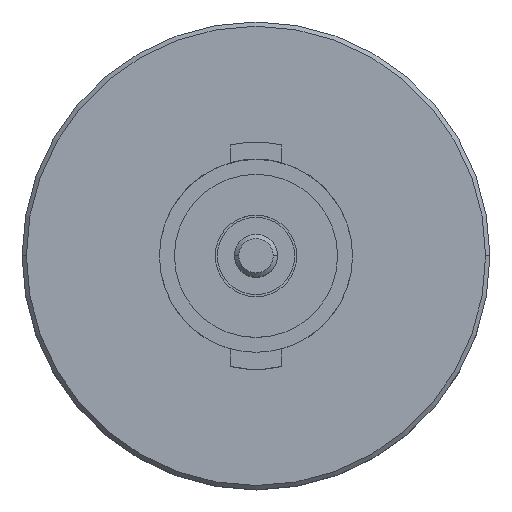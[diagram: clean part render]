
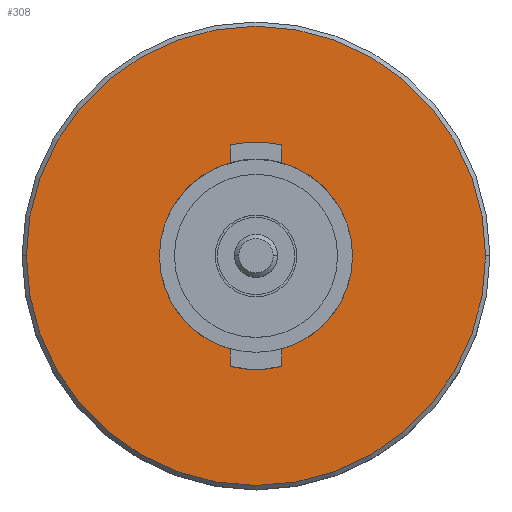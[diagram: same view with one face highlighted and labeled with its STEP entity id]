
A CAD part, top view. The second image highlights one B-rep face of the part: STEP entity #308.
In plain terms, the highlighted planar face has unit normal (0, 0, 1).
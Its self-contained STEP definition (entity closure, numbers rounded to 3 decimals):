
#24 = VECTOR ( 'NONE', #396, 1000. ) ;
#30 = DIRECTION ( 'NONE',  ( 0., 0., 1. ) ) ;
#41 = EDGE_CURVE ( 'NONE', #1158, #607, #622, .T. ) ;
#80 = AXIS2_PLACEMENT_3D ( 'NONE', #1608, #30, #760 ) ;
#83 = ORIENTED_EDGE ( 'NONE', *, *, #1763, .F. ) ;
#91 = CIRCLE ( 'NONE', #80, 2.25 ) ;
#105 = DIRECTION ( 'NONE',  ( -0.267, 0.964, 0. ) ) ;
#125 = AXIS2_PLACEMENT_3D ( 'NONE', #387, #1079, #1749 ) ;
#137 = EDGE_CURVE ( 'NONE', #607, #1485, #1885, .T. ) ;
#153 = VERTEX_POINT ( 'NONE', #1266 ) ;
#205 = CIRCLE ( 'NONE', #125, 2.25 ) ;
#216 = AXIS2_PLACEMENT_3D ( 'NONE', #491, #1185, #1853 ) ;
#240 = CARTESIAN_POINT ( 'NONE',  ( 20., 0., 30. ) ) ;
#242 = LINE ( 'NONE', #950, #2121 ) ;
#244 = EDGE_CURVE ( 'NONE', #1871, #1463, #91, .T. ) ;
#308 = ADVANCED_FACE ( 'NONE', ( #430, #1120 ), #1789, .T. ) ;
#329 = DIRECTION ( 'NONE',  ( -1., 0., 0. ) ) ;
#339 = AXIS2_PLACEMENT_3D ( 'NONE', #240, #948, #1626 ) ;
#360 = CARTESIAN_POINT ( 'NONE',  ( 19.4, 2.581, 30. ) ) ;
#381 = ORIENTED_EDGE ( 'NONE', *, *, #2131, .F. ) ;
#387 = CARTESIAN_POINT ( 'NONE',  ( 20., 0., 30. ) ) ;
#396 = DIRECTION ( 'NONE',  ( 0., -1., 0. ) ) ;
#401 = DIRECTION ( 'NONE',  ( 0., 0., 1. ) ) ;
#430 = FACE_OUTER_BOUND ( 'NONE', #1325, .T. ) ;
#490 = CARTESIAN_POINT ( 'NONE',  ( 20.6, -2.581, 30. ) ) ;
#491 = CARTESIAN_POINT ( 'NONE',  ( 20., 0., 30. ) ) ;
#494 = CARTESIAN_POINT ( 'NONE',  ( 20., 0., 30. ) ) ;
#519 = VECTOR ( 'NONE', #2179, 1000. ) ;
#534 = VERTEX_POINT ( 'NONE', #1863 ) ;
#582 = VECTOR ( 'NONE', #1054, 1000. ) ;
#607 = VERTEX_POINT ( 'NONE', #1567 ) ;
#620 = ORIENTED_EDGE ( 'NONE', *, *, #1744, .F. ) ;
#622 = CIRCLE ( 'NONE', #216, 2.65 ) ;
#674 = AXIS2_PLACEMENT_3D ( 'NONE', #1566, #2226, #710 ) ;
#710 = DIRECTION ( 'NONE',  ( 1., 0., 0. ) ) ;
#720 = ORIENTED_EDGE ( 'NONE', *, *, #1078, .F. ) ;
#730 = AXIS2_PLACEMENT_3D ( 'NONE', #1195, #1861, #329 ) ;
#750 = CARTESIAN_POINT ( 'NONE',  ( 14.65, 0., 30. ) ) ;
#760 = DIRECTION ( 'NONE',  ( -1., 0., 0. ) ) ;
#785 = CIRCLE ( 'NONE', #823, 5.35 ) ;
#823 = AXIS2_PLACEMENT_3D ( 'NONE', #1921, #401, #1092 ) ;
#834 = LINE ( 'NONE', #1522, #519 ) ;
#946 = CARTESIAN_POINT ( 'NONE',  ( 17.75, 0., 30. ) ) ;
#948 = DIRECTION ( 'NONE',  ( 0., 0., 1. ) ) ;
#950 = CARTESIAN_POINT ( 'NONE',  ( 20.6, -2.581, 30. ) ) ;
#955 = VERTEX_POINT ( 'NONE', #1253 ) ;
#989 = ORIENTED_EDGE ( 'NONE', *, *, #1480, .F. ) ;
#993 = ORIENTED_EDGE ( 'NONE', *, *, #244, .F. ) ;
#995 = CARTESIAN_POINT ( 'NONE',  ( 20., 0., 30. ) ) ;
#1054 = DIRECTION ( 'NONE',  ( 0., -1., 0. ) ) ;
#1078 = EDGE_CURVE ( 'NONE', #2041, #153, #242, .T. ) ;
#1079 = DIRECTION ( 'NONE',  ( 0., 0., 1. ) ) ;
#1092 = DIRECTION ( 'NONE',  ( 1., 0., 0. ) ) ;
#1120 = FACE_BOUND ( 'NONE', #1991, .T. ) ;
#1148 = ORIENTED_EDGE ( 'NONE', *, *, #1275, .T. ) ;
#1158 = VERTEX_POINT ( 'NONE', #1994 ) ;
#1185 = DIRECTION ( 'NONE',  ( 0., 0., 1. ) ) ;
#1188 = CARTESIAN_POINT ( 'NONE',  ( 19.4, 2.169, 30. ) ) ;
#1189 = DIRECTION ( 'NONE',  ( 0., 0., 1. ) ) ;
#1195 = CARTESIAN_POINT ( 'NONE',  ( 20., 0., 30. ) ) ;
#1200 = CIRCLE ( 'NONE', #674, 2.25 ) ;
#1221 = EDGE_CURVE ( 'NONE', #955, #2041, #1368, .T. ) ;
#1253 = CARTESIAN_POINT ( 'NONE',  ( 19.4, -2.581, 30. ) ) ;
#1258 = LINE ( 'NONE', #1918, #24 ) ;
#1266 = CARTESIAN_POINT ( 'NONE',  ( 20.6, -2.169, 30. ) ) ;
#1275 = EDGE_CURVE ( 'NONE', #2245, #1655, #785, .T. ) ;
#1305 = CARTESIAN_POINT ( 'NONE',  ( 25.35, 0., 30. ) ) ;
#1325 = EDGE_LOOP ( 'NONE', ( #2008, #1148 ) ) ;
#1368 = CIRCLE ( 'NONE', #1404, 2.65 ) ;
#1404 = AXIS2_PLACEMENT_3D ( 'NONE', #494, #1189, #1856 ) ;
#1446 = EDGE_CURVE ( 'NONE', #1485, #1871, #1661, .T. ) ;
#1463 = VERTEX_POINT ( 'NONE', #2002 ) ;
#1480 = EDGE_CURVE ( 'NONE', #1505, #1158, #834, .T. ) ;
#1485 = VERTEX_POINT ( 'NONE', #1188 ) ;
#1505 = VERTEX_POINT ( 'NONE', #2193 ) ;
#1522 = CARTESIAN_POINT ( 'NONE',  ( 20.6, 2.169, 30. ) ) ;
#1566 = CARTESIAN_POINT ( 'NONE',  ( 20., 0., 30. ) ) ;
#1567 = CARTESIAN_POINT ( 'NONE',  ( 19.4, 2.581, 30. ) ) ;
#1581 = ORIENTED_EDGE ( 'NONE', *, *, #41, .F. ) ;
#1608 = CARTESIAN_POINT ( 'NONE',  ( 20., 0., 30. ) ) ;
#1626 = DIRECTION ( 'NONE',  ( 1., 0., 0. ) ) ;
#1631 = DIRECTION ( 'NONE',  ( 0., 1., 0. ) ) ;
#1655 = VERTEX_POINT ( 'NONE', #750 ) ;
#1661 = CIRCLE ( 'NONE', #1768, 2.25 ) ;
#1670 = DIRECTION ( 'NONE',  ( 0., 0., 1. ) ) ;
#1693 = CIRCLE ( 'NONE', #730, 5.35 ) ;
#1744 = EDGE_CURVE ( 'NONE', #153, #534, #205, .T. ) ;
#1749 = DIRECTION ( 'NONE',  ( 0.267, -0.964, 0. ) ) ;
#1763 = EDGE_CURVE ( 'NONE', #1463, #955, #1258, .T. ) ;
#1768 = AXIS2_PLACEMENT_3D ( 'NONE', #995, #1670, #105 ) ;
#1789 = PLANE ( 'NONE',  #339 ) ;
#1853 = DIRECTION ( 'NONE',  ( 0., 1., 0. ) ) ;
#1856 = DIRECTION ( 'NONE',  ( -0.226, -0.974, 0. ) ) ;
#1861 = DIRECTION ( 'NONE',  ( 0., 0., 1. ) ) ;
#1863 = CARTESIAN_POINT ( 'NONE',  ( 22.25, 0., 30. ) ) ;
#1871 = VERTEX_POINT ( 'NONE', #946 ) ;
#1885 = LINE ( 'NONE', #360, #582 ) ;
#1918 = CARTESIAN_POINT ( 'NONE',  ( 19.4, -2.169, 30. ) ) ;
#1921 = CARTESIAN_POINT ( 'NONE',  ( 20., 0., 30. ) ) ;
#1934 = ORIENTED_EDGE ( 'NONE', *, *, #1221, .F. ) ;
#1991 = EDGE_LOOP ( 'NONE', ( #1581, #989, #381, #620, #720, #1934, #83, #993, #2200, #2053 ) ) ;
#1994 = CARTESIAN_POINT ( 'NONE',  ( 20.6, 2.581, 30. ) ) ;
#2002 = CARTESIAN_POINT ( 'NONE',  ( 19.4, -2.169, 30. ) ) ;
#2008 = ORIENTED_EDGE ( 'NONE', *, *, #2076, .T. ) ;
#2041 = VERTEX_POINT ( 'NONE', #490 ) ;
#2053 = ORIENTED_EDGE ( 'NONE', *, *, #137, .F. ) ;
#2076 = EDGE_CURVE ( 'NONE', #1655, #2245, #1693, .T. ) ;
#2121 = VECTOR ( 'NONE', #1631, 1000. ) ;
#2131 = EDGE_CURVE ( 'NONE', #534, #1505, #1200, .T. ) ;
#2179 = DIRECTION ( 'NONE',  ( 0., 1., 0. ) ) ;
#2193 = CARTESIAN_POINT ( 'NONE',  ( 20.6, 2.169, 30. ) ) ;
#2200 = ORIENTED_EDGE ( 'NONE', *, *, #1446, .F. ) ;
#2226 = DIRECTION ( 'NONE',  ( 0., 0., 1. ) ) ;
#2245 = VERTEX_POINT ( 'NONE', #1305 ) ;
